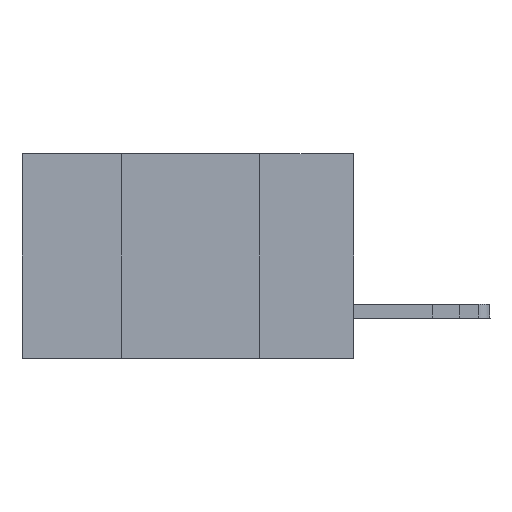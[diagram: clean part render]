
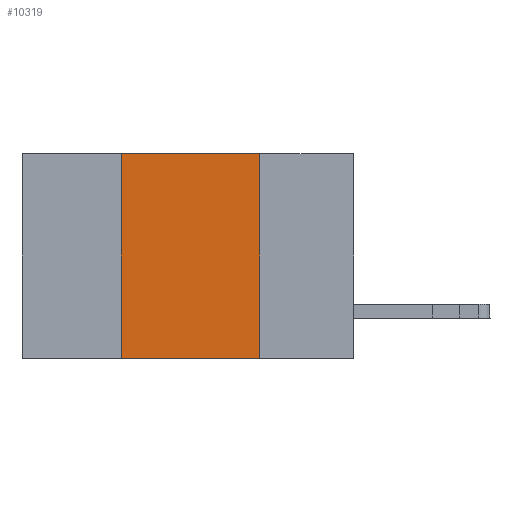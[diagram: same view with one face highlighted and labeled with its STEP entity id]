
A CAD part, left-side view. The second image highlights one B-rep face of the part: STEP entity #10319.
In plain terms, the highlighted planar face has unit normal (-1, 0, 0).
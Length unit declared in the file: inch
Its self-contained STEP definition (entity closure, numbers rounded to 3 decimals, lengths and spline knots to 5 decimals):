
#217 = LINE ( 'NONE', #598, #8957 ) ;
#598 = CARTESIAN_POINT ( 'NONE',  ( 0., 0.17, 0. ) ) ;
#2746 = VERTEX_POINT ( 'NONE', #9900 ) ;
#2992 = ORIENTED_EDGE ( 'NONE', *, *, #4757, .F. ) ;
#3094 = CARTESIAN_POINT ( 'NONE',  ( 0., 0.6, 0. ) ) ;
#3104 = ORIENTED_EDGE ( 'NONE', *, *, #4819, .F. ) ;
#3724 = AXIS2_PLACEMENT_3D ( 'NONE', #3094, #8879, #4343 ) ;
#4066 = LINE ( 'NONE', #4162, #17353 ) ;
#4162 = CARTESIAN_POINT ( 'NONE',  ( 0., 0.6, 0. ) ) ;
#4341 = CARTESIAN_POINT ( 'NONE',  ( 0., 0.6, -0.37 ) ) ;
#4343 = DIRECTION ( 'NONE',  ( 0., 0., -1. ) ) ;
#4757 = EDGE_CURVE ( 'NONE', #2746, #10814, #217, .T. ) ;
#4819 = EDGE_CURVE ( 'NONE', #11407, #6648, #9410, .T. ) ;
#5046 = VECTOR ( 'NONE', #8253, 39.37008 ) ;
#5604 = VECTOR ( 'NONE', #10085, 39.37008 ) ;
#6376 = DIRECTION ( 'NONE',  ( 0., 0., -1. ) ) ;
#6648 = VERTEX_POINT ( 'NONE', #7703 ) ;
#6827 = CARTESIAN_POINT ( 'NONE',  ( 0., 0.42, -0.37 ) ) ;
#7703 = CARTESIAN_POINT ( 'NONE',  ( 0., 0.42, 0. ) ) ;
#8253 = DIRECTION ( 'NONE',  ( 0., 0., 1. ) ) ;
#8594 = FACE_OUTER_BOUND ( 'NONE', #14731, .T. ) ;
#8879 = DIRECTION ( 'NONE',  ( 1., 0., 0. ) ) ;
#8957 = VECTOR ( 'NONE', #6376, 39.37008 ) ;
#9410 = LINE ( 'NONE', #12139, #5046 ) ;
#9739 = DIRECTION ( 'NONE',  ( 0., -1., 0. ) ) ;
#9900 = CARTESIAN_POINT ( 'NONE',  ( 0., 0.17, 0. ) ) ;
#10085 = DIRECTION ( 'NONE',  ( 0., -1., 0. ) ) ;
#10319 = ADVANCED_FACE ( 'NONE', ( #8594 ), #14382, .F. ) ;
#10627 = CARTESIAN_POINT ( 'NONE',  ( 0., 0.17, -0.37 ) ) ;
#10814 = VERTEX_POINT ( 'NONE', #10627 ) ;
#11407 = VERTEX_POINT ( 'NONE', #6827 ) ;
#11519 = LINE ( 'NONE', #4341, #5604 ) ;
#12139 = CARTESIAN_POINT ( 'NONE',  ( 0., 0.42, 0. ) ) ;
#14299 = ORIENTED_EDGE ( 'NONE', *, *, #14876, .F. ) ;
#14382 = PLANE ( 'NONE',  #3724 ) ;
#14731 = EDGE_LOOP ( 'NONE', ( #2992, #14299, #3104, #15119 ) ) ;
#14876 = EDGE_CURVE ( 'NONE', #6648, #2746, #4066, .T. ) ;
#15092 = EDGE_CURVE ( 'NONE', #11407, #10814, #11519, .T. ) ;
#15119 = ORIENTED_EDGE ( 'NONE', *, *, #15092, .T. ) ;
#17353 = VECTOR ( 'NONE', #9739, 39.37008 ) ;
